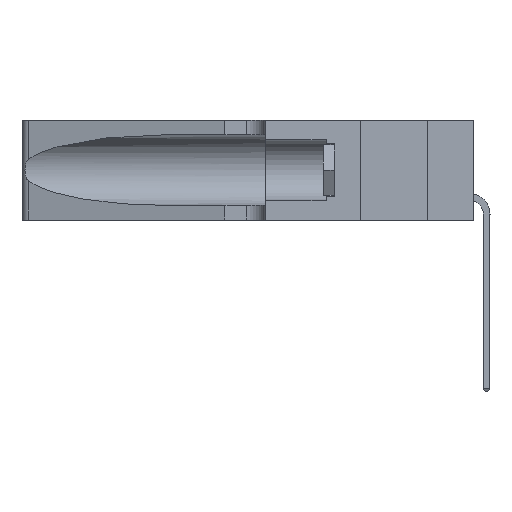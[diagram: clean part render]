
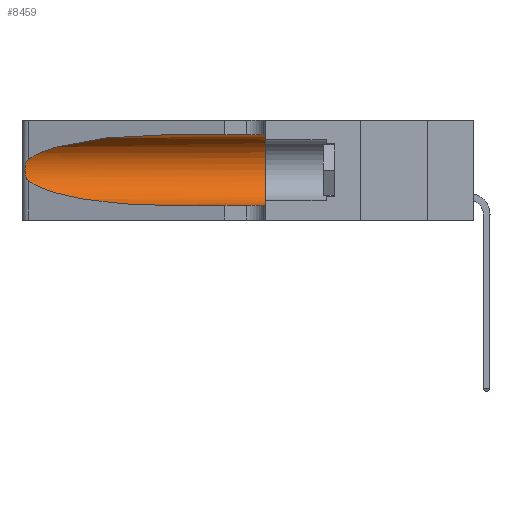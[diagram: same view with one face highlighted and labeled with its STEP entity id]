
A CAD part, left-side view. The second image highlights one B-rep face of the part: STEP entity #8459.
In plain terms, the highlighted cylindrical face has radius 3.308 mm (diameter 6.617 mm), a partial arc.
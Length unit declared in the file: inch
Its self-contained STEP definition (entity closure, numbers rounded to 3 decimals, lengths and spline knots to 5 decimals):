
#15 = CARTESIAN_POINT ( 'NONE',  ( 0.25854, 1.2359, 0.20912 ) ) ;
#508 = CARTESIAN_POINT ( 'NONE',  ( 0.25555, 1.22993, 0.14849 ) ) ;
#987 = ORIENTED_EDGE ( 'NONE', *, *, #41425, .F. ) ;
#1359 = EDGE_CURVE ( 'NONE', #19174, #8378, #27747, .T. ) ;
#1455 = CARTESIAN_POINT ( 'NONE',  ( 0.2373, 1.15595, 0.08982 ) ) ;
#1800 = CARTESIAN_POINT ( 'NONE',  ( 0.25487, 1.22718, 0.14631 ) ) ;
#1847 = EDGE_CURVE ( 'NONE', #8378, #28190, #8325, .T. ) ;
#2719 = VERTEX_POINT ( 'NONE', #28165 ) ;
#3018 = ORIENTED_EDGE ( 'NONE', *, *, #1359, .T. ) ;
#5028 = CARTESIAN_POINT ( 'NONE',  ( 0.18966, 0.96281, 0.05475 ) ) ;
#5522 = CARTESIAN_POINT ( 'NONE',  ( 0.1305, 0.72297, 0.05475 ) ) ;
#5681 = CARTESIAN_POINT ( 'NONE',  ( 0.1305, 0.72297, 0.31525 ) ) ;
#6360 = VERTEX_POINT ( 'NONE', #37603 ) ;
#6448 = CARTESIAN_POINT ( 'NONE',  ( 0.1305, 0.72297, 0.05475 ) ) ;
#6639 = CARTESIAN_POINT ( 'NONE',  ( 0.18966, 0.96281, 0.31525 ) ) ;
#6997 = LINE ( 'NONE', #46441, #36882 ) ;
#7128 = CARTESIAN_POINT ( 'NONE',  ( 0.1305, 0.35, 0.185 ) ) ;
#7851 = EDGE_LOOP ( 'NONE', ( #3018, #10888, #10110, #28713, #29937, #987 ) ) ;
#8175 = CARTESIAN_POINT ( 'NONE',  ( 0.25487, 1.22718, 0.14631 ) ) ;
#8325 = B_SPLINE_CURVE_WITH_KNOTS ( 'NONE', 3,
 ( #17046, #10919, #18257, #31074, #15, #43196, #46983, #34998, #15533, #27634, #16519, #20123, #508, #8175 ),
 .UNSPECIFIED., .F., .F.,
 ( 4, 2, 2, 2, 2, 2, 4 ),
 ( 0., 0.00027, 0.00053, 0.00107, 0.0016, 0.00187, 0.00214 ),
 .UNSPECIFIED. ) ;
#8378 = VERTEX_POINT ( 'NONE', #46335 ) ;
#8459 = ADVANCED_FACE ( 'NONE', ( #22795 ), #22178, .F. ) ;
#10110 = ORIENTED_EDGE ( 'NONE', *, *, #20754, .T. ) ;
#10888 = ORIENTED_EDGE ( 'NONE', *, *, #1847, .T. ) ;
#10919 = CARTESIAN_POINT ( 'NONE',  ( 0.25555, 1.22994, 0.2215 ) ) ;
#11053 = DIRECTION ( 'NONE',  ( 0., 1., 0. ) ) ;
#11150 = EDGE_CURVE ( 'NONE', #2719, #6360, #17849, .T. ) ;
#14121 = CARTESIAN_POINT ( 'NONE',  ( 0.25487, 1.22718, 0.14631 ) ) ;
#15533 = CARTESIAN_POINT ( 'NONE',  ( 0.26017, 1.23833, 0.17102 ) ) ;
#16088 = VERTEX_POINT ( 'NONE', #6448 ) ;
#16519 = CARTESIAN_POINT ( 'NONE',  ( 0.25789, 1.23486, 0.15765 ) ) ;
#17046 = CARTESIAN_POINT ( 'NONE',  ( 0.25487, 1.22718, 0.22369 ) ) ;
#17849 = CIRCLE ( 'NONE', #21383, 0.13025 ) ;
#18257 = CARTESIAN_POINT ( 'NONE',  ( 0.25639, 1.23184, 0.21858 ) ) ;
#18357 = VECTOR ( 'NONE', #43873, 39.37008 ) ;
#19174 = VERTEX_POINT ( 'NONE', #5681 ) ;
#20123 = CARTESIAN_POINT ( 'NONE',  ( 0.25639, 1.23186, 0.15144 ) ) ;
#20754 = EDGE_CURVE ( 'NONE', #28190, #16088, #33489, .T. ) ;
#21383 = AXIS2_PLACEMENT_3D ( 'NONE', #7128, #11053, #27093 ) ;
#22178 = CYLINDRICAL_SURFACE ( 'NONE', #31806, 0.13025 ) ;
#22795 = FACE_OUTER_BOUND ( 'NONE', #7851, .T. ) ;
#23485 = DIRECTION ( 'NONE',  ( 0., -1., 0. ) ) ;
#27093 = DIRECTION ( 'NONE',  ( 0., 0., 1. ) ) ;
#27634 = CARTESIAN_POINT ( 'NONE',  ( 0.25856, 1.23593, 0.16098 ) ) ;
#27747 =( BOUNDED_CURVE ( )  B_SPLINE_CURVE ( 3, ( #33773, #6639, #49582, #29349 ),
 .UNSPECIFIED., .F., .F. ) 
 B_SPLINE_CURVE_WITH_KNOTS ( ( 4, 4 ),
 ( 1.5708, 2.84003 ),
 .UNSPECIFIED. ) 
 CURVE ( )  GEOMETRIC_REPRESENTATION_ITEM ( )  RATIONAL_B_SPLINE_CURVE ( ( 1., 0.87, 0.87, 1. ) ) 
 REPRESENTATION_ITEM ( '' )  );
#28165 = CARTESIAN_POINT ( 'NONE',  ( 0.1305, 0.35, 0.31525 ) ) ;
#28190 = VERTEX_POINT ( 'NONE', #14121 ) ;
#28713 = ORIENTED_EDGE ( 'NONE', *, *, #38370, .T. ) ;
#29349 = CARTESIAN_POINT ( 'NONE',  ( 0.25487, 1.22718, 0.22369 ) ) ;
#29937 = ORIENTED_EDGE ( 'NONE', *, *, #11150, .F. ) ;
#30695 = DIRECTION ( 'NONE',  ( 0., -1., 0. ) ) ;
#31074 = CARTESIAN_POINT ( 'NONE',  ( 0.25787, 1.23484, 0.2124 ) ) ;
#31806 = AXIS2_PLACEMENT_3D ( 'NONE', #46403, #23485, #50526 ) ;
#31929 = CARTESIAN_POINT ( 'NONE',  ( 0.1305, 1.61858, 0.05475 ) ) ;
#33489 =( BOUNDED_CURVE ( )  B_SPLINE_CURVE ( 3, ( #1800, #1455, #5028, #5522 ),
 .UNSPECIFIED., .F., .F. ) 
 B_SPLINE_CURVE_WITH_KNOTS ( ( 4, 4 ),
 ( 3.44316, 4.71239 ),
 .UNSPECIFIED. ) 
 CURVE ( )  GEOMETRIC_REPRESENTATION_ITEM ( )  RATIONAL_B_SPLINE_CURVE ( ( 1., 0.87, 0.87, 1. ) ) 
 REPRESENTATION_ITEM ( '' )  );
#33773 = CARTESIAN_POINT ( 'NONE',  ( 0.1305, 0.72297, 0.31525 ) ) ;
#34998 = CARTESIAN_POINT ( 'NONE',  ( 0.26075, 1.23896, 0.178 ) ) ;
#36882 = VECTOR ( 'NONE', #30695, 39.37008 ) ;
#37603 = CARTESIAN_POINT ( 'NONE',  ( 0.1305, 0.35, 0.05475 ) ) ;
#38370 = EDGE_CURVE ( 'NONE', #16088, #6360, #44047, .T. ) ;
#41425 = EDGE_CURVE ( 'NONE', #19174, #2719, #6997, .T. ) ;
#43196 = CARTESIAN_POINT ( 'NONE',  ( 0.26018, 1.23835, 0.19895 ) ) ;
#43873 = DIRECTION ( 'NONE',  ( 0., -1., 0. ) ) ;
#44047 = LINE ( 'NONE', #31929, #18357 ) ;
#46335 = CARTESIAN_POINT ( 'NONE',  ( 0.25487, 1.22718, 0.22369 ) ) ;
#46403 = CARTESIAN_POINT ( 'NONE',  ( 0.1305, 1.61858, 0.185 ) ) ;
#46441 = CARTESIAN_POINT ( 'NONE',  ( 0.1305, 1.61858, 0.31525 ) ) ;
#46983 = CARTESIAN_POINT ( 'NONE',  ( 0.26075, 1.23896, 0.19203 ) ) ;
#49582 = CARTESIAN_POINT ( 'NONE',  ( 0.2373, 1.15595, 0.28018 ) ) ;
#50526 = DIRECTION ( 'NONE',  ( 0., 0., -1. ) ) ;
